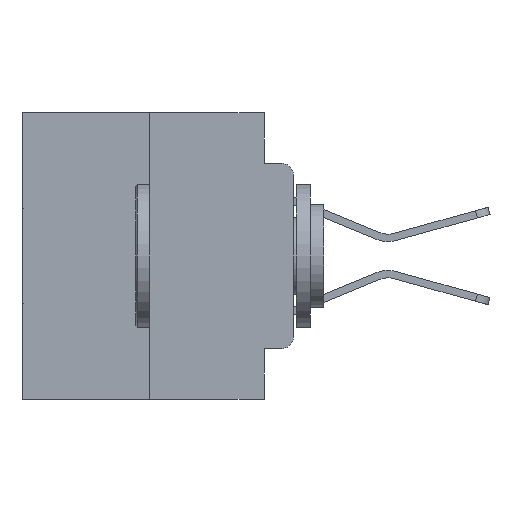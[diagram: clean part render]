
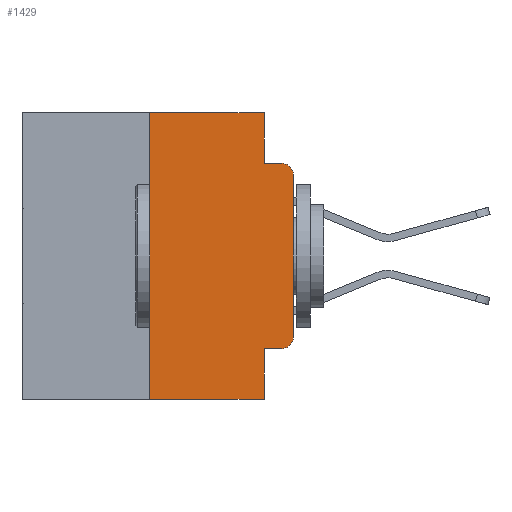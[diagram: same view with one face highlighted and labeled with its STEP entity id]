
A CAD part, left-side view. The second image highlights one B-rep face of the part: STEP entity #1429.
In plain terms, the highlighted planar face has unit normal (-1, 0, 0).
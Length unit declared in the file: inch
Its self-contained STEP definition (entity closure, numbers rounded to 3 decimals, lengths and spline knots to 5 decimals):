
#486 = VERTEX_POINT ( 'NONE', #12634 ) ;
#1160 = ORIENTED_EDGE ( 'NONE', *, *, #17562, .T. ) ;
#1429 = ADVANCED_FACE ( 'NONE', ( #29281 ), #26870, .F. ) ;
#1842 = EDGE_CURVE ( 'NONE', #26916, #3439, #22297, .T. ) ;
#2061 = LINE ( 'NONE', #11263, #3939 ) ;
#2214 = VECTOR ( 'NONE', #3138, 39.37008 ) ;
#2255 = DIRECTION ( 'NONE',  ( 0., 0., -1. ) ) ;
#2755 = EDGE_CURVE ( 'NONE', #15285, #21055, #17737, .T. ) ;
#2841 = CARTESIAN_POINT ( 'NONE',  ( 0., 0.051, -0.4115 ) ) ;
#3138 = DIRECTION ( 'NONE',  ( 0., -1., 0. ) ) ;
#3262 = CARTESIAN_POINT ( 'NONE',  ( 0., 0.051, -0.5 ) ) ;
#3381 = ORIENTED_EDGE ( 'NONE', *, *, #26682, .F. ) ;
#3439 = VERTEX_POINT ( 'NONE', #14993 ) ;
#3545 = CARTESIAN_POINT ( 'NONE',  ( 0., 0.25, 0. ) ) ;
#3726 = ORIENTED_EDGE ( 'NONE', *, *, #11894, .T. ) ;
#3749 = CARTESIAN_POINT ( 'NONE',  ( 0., 0.051, -0.4115 ) ) ;
#3754 = AXIS2_PLACEMENT_3D ( 'NONE', #6537, #15625, #4160 ) ;
#3939 = VECTOR ( 'NONE', #13655, 39.37008 ) ;
#4160 = DIRECTION ( 'NONE',  ( 0., 0., -1. ) ) ;
#4810 = AXIS2_PLACEMENT_3D ( 'NONE', #17647, #26225, #28620 ) ;
#5318 = DIRECTION ( 'NONE',  ( 0., 0., 1. ) ) ;
#5417 = CARTESIAN_POINT ( 'NONE',  ( 0., 0., -0.3915 ) ) ;
#5673 = DIRECTION ( 'NONE',  ( 0., -1., 0. ) ) ;
#5745 = VERTEX_POINT ( 'NONE', #16985 ) ;
#6108 = CARTESIAN_POINT ( 'NONE',  ( 0., 0.473, -0.5 ) ) ;
#6266 = DIRECTION ( 'NONE',  ( -1., 0., 0. ) ) ;
#6537 = CARTESIAN_POINT ( 'NONE',  ( 0., 0.473, 0. ) ) ;
#6618 = VECTOR ( 'NONE', #13520, 39.37008 ) ;
#6760 = EDGE_CURVE ( 'NONE', #5745, #3439, #9620, .T. ) ;
#8132 = DIRECTION ( 'NONE',  ( 0., -1., 0. ) ) ;
#8289 = EDGE_CURVE ( 'NONE', #22470, #26916, #8974, .T. ) ;
#8782 = CARTESIAN_POINT ( 'NONE',  ( 0., 0.02, -0.3915 ) ) ;
#8914 = VERTEX_POINT ( 'NONE', #17297 ) ;
#8974 = LINE ( 'NONE', #15705, #23502 ) ;
#9620 = CIRCLE ( 'NONE', #4810, 0.02 ) ;
#9926 = CIRCLE ( 'NONE', #13770, 0.02 ) ;
#9975 = VERTEX_POINT ( 'NONE', #23274 ) ;
#10728 = DIRECTION ( 'NONE',  ( 0., 0., -1. ) ) ;
#10808 = EDGE_CURVE ( 'NONE', #15285, #486, #11754, .T. ) ;
#11263 = CARTESIAN_POINT ( 'NONE',  ( 0., 0., 0. ) ) ;
#11271 = CARTESIAN_POINT ( 'NONE',  ( 0., 0.051, -0.0885 ) ) ;
#11373 = VERTEX_POINT ( 'NONE', #5417 ) ;
#11754 = LINE ( 'NONE', #2841, #2214 ) ;
#11894 = EDGE_CURVE ( 'NONE', #8914, #21055, #28564, .T. ) ;
#12156 = ORIENTED_EDGE ( 'NONE', *, *, #8289, .F. ) ;
#12205 = VECTOR ( 'NONE', #8132, 39.37008 ) ;
#12634 = CARTESIAN_POINT ( 'NONE',  ( 0., 0.02, -0.4115 ) ) ;
#13392 = EDGE_LOOP ( 'NONE', ( #24087, #23539, #14390, #12156, #3381, #15258, #3726, #22966, #17944, #1160 ) ) ;
#13520 = DIRECTION ( 'NONE',  ( 0., -1., 0. ) ) ;
#13655 = DIRECTION ( 'NONE',  ( 0., 0., 1. ) ) ;
#13770 = AXIS2_PLACEMENT_3D ( 'NONE', #8782, #6266, #10728 ) ;
#14390 = ORIENTED_EDGE ( 'NONE', *, *, #1842, .F. ) ;
#14715 = LINE ( 'NONE', #14857, #12205 ) ;
#14857 = CARTESIAN_POINT ( 'NONE',  ( 0., 0.473, 0. ) ) ;
#14993 = CARTESIAN_POINT ( 'NONE',  ( 0., 0.02, -0.0885 ) ) ;
#15258 = ORIENTED_EDGE ( 'NONE', *, *, #23262, .F. ) ;
#15285 = VERTEX_POINT ( 'NONE', #3749 ) ;
#15625 = DIRECTION ( 'NONE',  ( 1., 0., 0. ) ) ;
#15705 = CARTESIAN_POINT ( 'NONE',  ( 0., 0.051, 0. ) ) ;
#16985 = CARTESIAN_POINT ( 'NONE',  ( 0., 0., -0.1085 ) ) ;
#17297 = CARTESIAN_POINT ( 'NONE',  ( 0., 0.25, -0.5 ) ) ;
#17562 = EDGE_CURVE ( 'NONE', #486, #11373, #9926, .T. ) ;
#17647 = CARTESIAN_POINT ( 'NONE',  ( 0., 0.02, -0.1085 ) ) ;
#17737 = LINE ( 'NONE', #17881, #28004 ) ;
#17881 = CARTESIAN_POINT ( 'NONE',  ( 0., 0.051, 0. ) ) ;
#17944 = ORIENTED_EDGE ( 'NONE', *, *, #10808, .T. ) ;
#21055 = VERTEX_POINT ( 'NONE', #3262 ) ;
#21244 = EDGE_CURVE ( 'NONE', #11373, #5745, #2061, .T. ) ;
#22297 = LINE ( 'NONE', #11271, #6618 ) ;
#22408 = VECTOR ( 'NONE', #5673, 39.37008 ) ;
#22470 = VERTEX_POINT ( 'NONE', #28450 ) ;
#22702 = DIRECTION ( 'NONE',  ( 0., 0., -1. ) ) ;
#22966 = ORIENTED_EDGE ( 'NONE', *, *, #2755, .F. ) ;
#23262 = EDGE_CURVE ( 'NONE', #8914, #9975, #25948, .T. ) ;
#23274 = CARTESIAN_POINT ( 'NONE',  ( 0., 0.25, 0. ) ) ;
#23502 = VECTOR ( 'NONE', #22702, 39.37008 ) ;
#23539 = ORIENTED_EDGE ( 'NONE', *, *, #6760, .T. ) ;
#24087 = ORIENTED_EDGE ( 'NONE', *, *, #21244, .T. ) ;
#25948 = LINE ( 'NONE', #3545, #28634 ) ;
#26225 = DIRECTION ( 'NONE',  ( -1., 0., 0. ) ) ;
#26682 = EDGE_CURVE ( 'NONE', #9975, #22470, #14715, .T. ) ;
#26870 = PLANE ( 'NONE',  #3754 ) ;
#26916 = VERTEX_POINT ( 'NONE', #28417 ) ;
#28004 = VECTOR ( 'NONE', #2255, 39.37008 ) ;
#28417 = CARTESIAN_POINT ( 'NONE',  ( 0., 0.051, -0.0885 ) ) ;
#28450 = CARTESIAN_POINT ( 'NONE',  ( 0., 0.051, 0. ) ) ;
#28564 = LINE ( 'NONE', #6108, #22408 ) ;
#28620 = DIRECTION ( 'NONE',  ( 0., 0., -1. ) ) ;
#28634 = VECTOR ( 'NONE', #5318, 39.37008 ) ;
#29281 = FACE_OUTER_BOUND ( 'NONE', #13392, .T. ) ;
